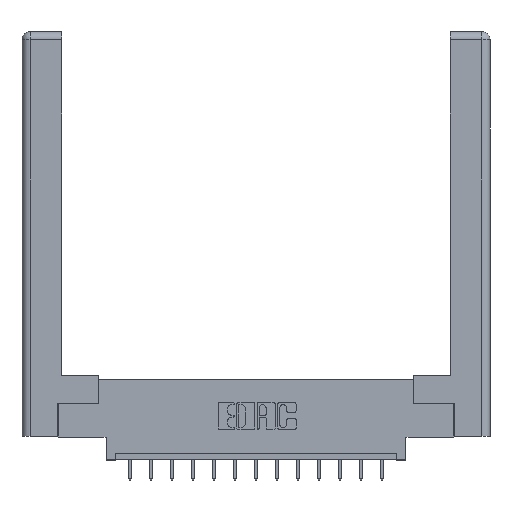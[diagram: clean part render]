
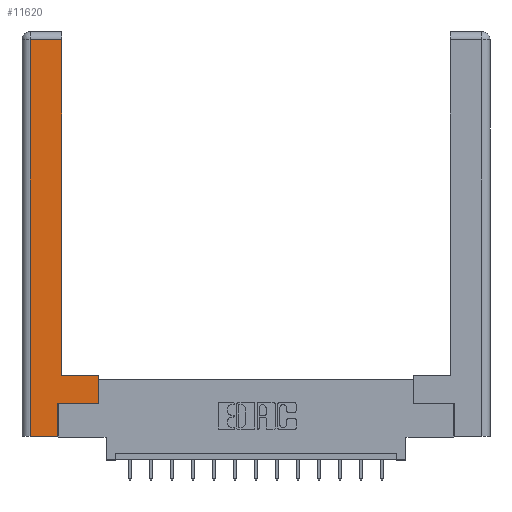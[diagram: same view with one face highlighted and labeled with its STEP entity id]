
A CAD part, top view. The second image highlights one B-rep face of the part: STEP entity #11620.
In plain terms, the highlighted planar face has unit normal (0, 0, 1).
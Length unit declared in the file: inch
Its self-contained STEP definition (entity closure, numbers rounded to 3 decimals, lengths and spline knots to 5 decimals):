
#81 = CARTESIAN_POINT ( 'NONE',  ( 0.265, 0.245, 0. ) ) ;
#86 = LINE ( 'NONE', #2435, #9110 ) ;
#108 = VECTOR ( 'NONE', #2503, 39.37008 ) ;
#246 = CARTESIAN_POINT ( 'NONE',  ( 0.295, 0.45, 0. ) ) ;
#329 = EDGE_CURVE ( 'NONE', #6763, #7069, #4452, .T. ) ;
#476 = CARTESIAN_POINT ( 'NONE',  ( 0.565, 0.45, 0. ) ) ;
#495 = ORIENTED_EDGE ( 'NONE', *, *, #7323, .T. ) ;
#1381 = VERTEX_POINT ( 'NONE', #14111 ) ;
#1438 = CARTESIAN_POINT ( 'NONE',  ( 0.265, 0., 0. ) ) ;
#1471 = VECTOR ( 'NONE', #13035, 39.37008 ) ;
#1490 = VECTOR ( 'NONE', #12609, 39.37008 ) ;
#1662 = VECTOR ( 'NONE', #14814, 39.37008 ) ;
#1919 = VECTOR ( 'NONE', #4392, 39.37008 ) ;
#2079 = LINE ( 'NONE', #11831, #11694 ) ;
#2435 = CARTESIAN_POINT ( 'NONE',  ( 0.0615, 2.94, 0. ) ) ;
#2444 = LINE ( 'NONE', #7592, #1490 ) ;
#2503 = DIRECTION ( 'NONE',  ( 0., -1., 0. ) ) ;
#2617 = VERTEX_POINT ( 'NONE', #14542 ) ;
#2686 = CARTESIAN_POINT ( 'NONE',  ( 0.265, 0., 0. ) ) ;
#3245 = VERTEX_POINT ( 'NONE', #476 ) ;
#3609 = ORIENTED_EDGE ( 'NONE', *, *, #7850, .T. ) ;
#3648 = CARTESIAN_POINT ( 'NONE',  ( 0.0615, 0., 0. ) ) ;
#3946 = DIRECTION ( 'NONE',  ( 1., 0., 0. ) ) ;
#4236 = CARTESIAN_POINT ( 'NONE',  ( 0.565, 0.45, 0. ) ) ;
#4392 = DIRECTION ( 'NONE',  ( 0., 1., 0. ) ) ;
#4452 = LINE ( 'NONE', #6637, #1919 ) ;
#4453 = CARTESIAN_POINT ( 'NONE',  ( 0., 0., 0. ) ) ;
#4747 = CARTESIAN_POINT ( 'NONE',  ( 0.565, 0.245, 0. ) ) ;
#4876 = VERTEX_POINT ( 'NONE', #246 ) ;
#5467 = DIRECTION ( 'NONE',  ( 0., 1., 0. ) ) ;
#5493 = DIRECTION ( 'NONE',  ( -1., 0., 0. ) ) ;
#5549 = CARTESIAN_POINT ( 'NONE',  ( 0.0615, 2.94, 0. ) ) ;
#6637 = CARTESIAN_POINT ( 'NONE',  ( 0.265, 0.245, 0. ) ) ;
#6698 = DIRECTION ( 'NONE',  ( 0., 0., -1. ) ) ;
#6763 = VERTEX_POINT ( 'NONE', #2686 ) ;
#6851 = EDGE_CURVE ( 'NONE', #4876, #1381, #2079, .T. ) ;
#6972 = VERTEX_POINT ( 'NONE', #3648 ) ;
#7044 = EDGE_CURVE ( 'NONE', #3245, #4876, #2444, .T. ) ;
#7069 = VERTEX_POINT ( 'NONE', #81 ) ;
#7323 = EDGE_CURVE ( 'NONE', #1381, #12546, #86, .T. ) ;
#7592 = CARTESIAN_POINT ( 'NONE',  ( 0.295, 0.45, 0. ) ) ;
#7850 = EDGE_CURVE ( 'NONE', #7069, #2617, #15129, .T. ) ;
#9110 = VECTOR ( 'NONE', #9899, 39.37008 ) ;
#9229 = ORIENTED_EDGE ( 'NONE', *, *, #13754, .T. ) ;
#9664 = ORIENTED_EDGE ( 'NONE', *, *, #6851, .T. ) ;
#9899 = DIRECTION ( 'NONE',  ( -1., 0., 0. ) ) ;
#10383 = FACE_OUTER_BOUND ( 'NONE', #12961, .T. ) ;
#10894 = ORIENTED_EDGE ( 'NONE', *, *, #329, .T. ) ;
#11592 = LINE ( 'NONE', #1438, #16056 ) ;
#11620 = ADVANCED_FACE ( 'NONE', ( #10383 ), #14309, .F. ) ;
#11694 = VECTOR ( 'NONE', #5467, 39.37008 ) ;
#11831 = CARTESIAN_POINT ( 'NONE',  ( 0.295, 3., 0. ) ) ;
#11856 = LINE ( 'NONE', #4236, #1471 ) ;
#11872 = LINE ( 'NONE', #12574, #108 ) ;
#12546 = VERTEX_POINT ( 'NONE', #5549 ) ;
#12574 = CARTESIAN_POINT ( 'NONE',  ( 0.0615, 0., 0. ) ) ;
#12609 = DIRECTION ( 'NONE',  ( -1., 0., 0. ) ) ;
#12961 = EDGE_LOOP ( 'NONE', ( #9664, #495, #13514, #15712, #10894, #3609, #9229, #15900 ) ) ;
#13035 = DIRECTION ( 'NONE',  ( 0., 1., 0. ) ) ;
#13438 = EDGE_CURVE ( 'NONE', #12546, #6972, #11872, .T. ) ;
#13514 = ORIENTED_EDGE ( 'NONE', *, *, #13438, .T. ) ;
#13754 = EDGE_CURVE ( 'NONE', #2617, #3245, #11856, .T. ) ;
#14111 = CARTESIAN_POINT ( 'NONE',  ( 0.295, 2.94, 0. ) ) ;
#14309 = PLANE ( 'NONE',  #14674 ) ;
#14542 = CARTESIAN_POINT ( 'NONE',  ( 0.565, 0.245, 0. ) ) ;
#14674 = AXIS2_PLACEMENT_3D ( 'NONE', #4453, #6698, #5493 ) ;
#14814 = DIRECTION ( 'NONE',  ( 1., 0., 0. ) ) ;
#15129 = LINE ( 'NONE', #4747, #1662 ) ;
#15551 = EDGE_CURVE ( 'NONE', #6972, #6763, #11592, .T. ) ;
#15712 = ORIENTED_EDGE ( 'NONE', *, *, #15551, .T. ) ;
#15900 = ORIENTED_EDGE ( 'NONE', *, *, #7044, .T. ) ;
#16056 = VECTOR ( 'NONE', #3946, 39.37008 ) ;
